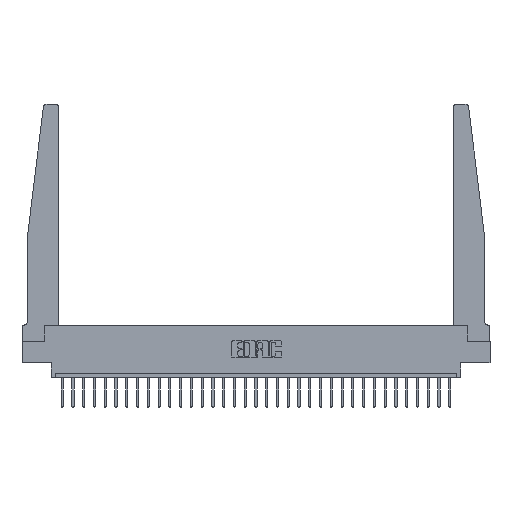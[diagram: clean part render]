
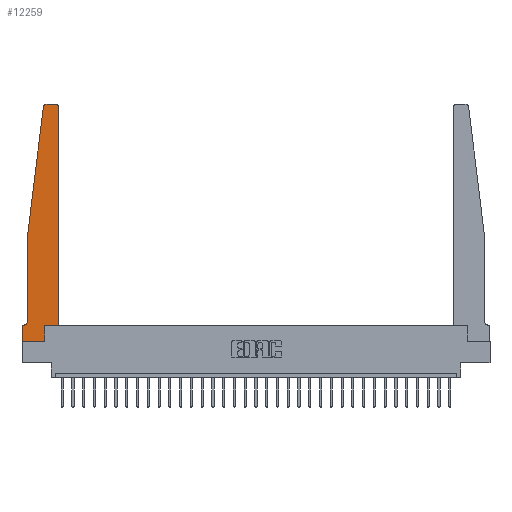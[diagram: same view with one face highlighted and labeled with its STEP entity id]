
A CAD part, top view. The second image highlights one B-rep face of the part: STEP entity #12259.
In plain terms, the highlighted planar face has unit normal (0, 0, 1).
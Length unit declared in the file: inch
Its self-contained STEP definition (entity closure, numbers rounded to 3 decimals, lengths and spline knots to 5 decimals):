
#752 = VERTEX_POINT ( 'NONE', #10985 ) ;
#1044 = CARTESIAN_POINT ( 'NONE',  ( 0.065, 1.25, 0.37 ) ) ;
#1066 = CARTESIAN_POINT ( 'NONE',  ( 0.2605, 0.18, 0.37 ) ) ;
#1808 = DIRECTION ( 'NONE',  ( 1., 0., 0. ) ) ;
#1950 = CARTESIAN_POINT ( 'NONE',  ( 0.395, 2.75, 0.37 ) ) ;
#2526 = DIRECTION ( 'NONE',  ( -1., 0., 0. ) ) ;
#2710 = ORIENTED_EDGE ( 'NONE', *, *, #28389, .T. ) ;
#3268 = CARTESIAN_POINT ( 'NONE',  ( 0.27653, 2.75, 0.37 ) ) ;
#3330 = VERTEX_POINT ( 'NONE', #6117 ) ;
#3364 = LINE ( 'NONE', #13726, #3900 ) ;
#3491 = CARTESIAN_POINT ( 'NONE',  ( 0.065, 0.2375, 0.37 ) ) ;
#3594 = CARTESIAN_POINT ( 'NONE',  ( 0.425, 0.18, 0.37 ) ) ;
#3679 = LINE ( 'NONE', #14845, #21138 ) ;
#3706 = EDGE_CURVE ( 'NONE', #10774, #10416, #12161, .T. ) ;
#3900 = VECTOR ( 'NONE', #22688, 39.37008 ) ;
#4049 = VECTOR ( 'NONE', #21246, 39.37008 ) ;
#4545 = CARTESIAN_POINT ( 'NONE',  ( 0.25, 2.75, 0.37 ) ) ;
#5401 = DIRECTION ( 'NONE',  ( 1., 0., 0. ) ) ;
#5425 = VERTEX_POINT ( 'NONE', #17508 ) ;
#5815 = ORIENTED_EDGE ( 'NONE', *, *, #12716, .T. ) ;
#6117 = CARTESIAN_POINT ( 'NONE',  ( 0.2605, 0.18, 0.37 ) ) ;
#6960 = ORIENTED_EDGE ( 'NONE', *, *, #20712, .T. ) ;
#7152 = VERTEX_POINT ( 'NONE', #1950 ) ;
#7187 = EDGE_CURVE ( 'NONE', #3330, #15897, #26473, .T. ) ;
#7619 = PLANE ( 'NONE',  #15195 ) ;
#7924 = CARTESIAN_POINT ( 'NONE',  ( 0.065, 1.25, 0.37 ) ) ;
#7941 = DIRECTION ( 'NONE',  ( -1., 0., 0. ) ) ;
#7980 = DIRECTION ( 'NONE',  ( 0., 1., 0. ) ) ;
#8244 = ORIENTED_EDGE ( 'NONE', *, *, #13116, .T. ) ;
#8629 = CARTESIAN_POINT ( 'NONE',  ( 0.27653, 2.72, 0.37 ) ) ;
#8886 = EDGE_CURVE ( 'NONE', #5425, #3330, #23819, .T. ) ;
#9019 = EDGE_CURVE ( 'NONE', #15897, #752, #21089, .T. ) ;
#9147 = VERTEX_POINT ( 'NONE', #22843 ) ;
#9743 = CARTESIAN_POINT ( 'NONE',  ( 0., 0., 0.37 ) ) ;
#9792 = ORIENTED_EDGE ( 'NONE', *, *, #3706, .T. ) ;
#10229 = CARTESIAN_POINT ( 'NONE',  ( 0.425, 0.18, 0.37 ) ) ;
#10416 = VERTEX_POINT ( 'NONE', #3491 ) ;
#10774 = VERTEX_POINT ( 'NONE', #15992 ) ;
#10856 = ORIENTED_EDGE ( 'NONE', *, *, #8886, .T. ) ;
#10985 = CARTESIAN_POINT ( 'NONE',  ( 0.425, 2.72, 0.37 ) ) ;
#11043 = CARTESIAN_POINT ( 'NONE',  ( 0.425, 0.18, 0.37 ) ) ;
#11393 = CIRCLE ( 'NONE', #27813, 0.05 ) ;
#11712 = AXIS2_PLACEMENT_3D ( 'NONE', #8629, #24461, #13454 ) ;
#12112 = DIRECTION ( 'NONE',  ( -1., 0., 0. ) ) ;
#12161 = LINE ( 'NONE', #7924, #4049 ) ;
#12259 = ADVANCED_FACE ( 'NONE', ( #27716 ), #7619, .T. ) ;
#12396 = VECTOR ( 'NONE', #24086, 39.37008 ) ;
#12489 = DIRECTION ( 'NONE',  ( 0., 0., 1. ) ) ;
#12716 = EDGE_CURVE ( 'NONE', #9147, #10774, #26163, .T. ) ;
#12717 = AXIS2_PLACEMENT_3D ( 'NONE', #23634, #12489, #23192 ) ;
#13116 = EDGE_CURVE ( 'NONE', #19179, #22123, #23379, .T. ) ;
#13243 = VECTOR ( 'NONE', #27735, 39.37008 ) ;
#13454 = DIRECTION ( 'NONE',  ( 1., 0., 0. ) ) ;
#13726 = CARTESIAN_POINT ( 'NONE',  ( 0., 0., 0.37 ) ) ;
#14601 = CIRCLE ( 'NONE', #12717, 0.03 ) ;
#14845 = CARTESIAN_POINT ( 'NONE',  ( 0.065, 0.1875, 0.37 ) ) ;
#15195 = AXIS2_PLACEMENT_3D ( 'NONE', #16525, #25500, #5401 ) ;
#15259 = VERTEX_POINT ( 'NONE', #3268 ) ;
#15888 = DIRECTION ( 'NONE',  ( 0., 0., -1. ) ) ;
#15897 = VERTEX_POINT ( 'NONE', #11043 ) ;
#15992 = CARTESIAN_POINT ( 'NONE',  ( 0.065, 1.25, 0.37 ) ) ;
#16525 = CARTESIAN_POINT ( 'NONE',  ( 0., 0.1875, 0.37 ) ) ;
#16642 = DIRECTION ( 'NONE',  ( 0., -1., 0. ) ) ;
#16828 = ORIENTED_EDGE ( 'NONE', *, *, #24704, .T. ) ;
#17469 = VECTOR ( 'NONE', #12112, 39.37008 ) ;
#17508 = CARTESIAN_POINT ( 'NONE',  ( 0.2605, 0., 0.37 ) ) ;
#17683 = VECTOR ( 'NONE', #1808, 39.37008 ) ;
#18280 = EDGE_LOOP ( 'NONE', ( #19956, #16828, #5815, #9792, #6960, #19572, #8244, #2710, #10856, #19670, #24414, #28059 ) ) ;
#18804 = EDGE_CURVE ( 'NONE', #752, #7152, #14601, .T. ) ;
#19150 = CARTESIAN_POINT ( 'NONE',  ( 0., 0., 0.37 ) ) ;
#19179 = VERTEX_POINT ( 'NONE', #22192 ) ;
#19572 = ORIENTED_EDGE ( 'NONE', *, *, #26651, .T. ) ;
#19670 = ORIENTED_EDGE ( 'NONE', *, *, #7187, .T. ) ;
#19956 = ORIENTED_EDGE ( 'NONE', *, *, #20917, .T. ) ;
#20264 = VERTEX_POINT ( 'NONE', #25290 ) ;
#20712 = EDGE_CURVE ( 'NONE', #10416, #20264, #11393, .T. ) ;
#20917 = EDGE_CURVE ( 'NONE', #7152, #15259, #27701, .T. ) ;
#21089 = LINE ( 'NONE', #10229, #13243 ) ;
#21138 = VECTOR ( 'NONE', #7941, 39.37008 ) ;
#21246 = DIRECTION ( 'NONE',  ( 0., -1., 0. ) ) ;
#22123 = VERTEX_POINT ( 'NONE', #19150 ) ;
#22192 = CARTESIAN_POINT ( 'NONE',  ( 0., 0.1875, 0.37 ) ) ;
#22688 = DIRECTION ( 'NONE',  ( 1., 0., 0. ) ) ;
#22843 = CARTESIAN_POINT ( 'NONE',  ( 0.24675, 2.72367, 0.37 ) ) ;
#23192 = DIRECTION ( 'NONE',  ( 1., 0., 0. ) ) ;
#23379 = LINE ( 'NONE', #9743, #28380 ) ;
#23634 = CARTESIAN_POINT ( 'NONE',  ( 0.395, 2.72, 0.37 ) ) ;
#23819 = LINE ( 'NONE', #1066, #24031 ) ;
#24031 = VECTOR ( 'NONE', #7980, 39.37008 ) ;
#24086 = DIRECTION ( 'NONE',  ( -0.122, -0.992, 0. ) ) ;
#24327 = CIRCLE ( 'NONE', #11712, 0.03 ) ;
#24414 = ORIENTED_EDGE ( 'NONE', *, *, #9019, .T. ) ;
#24461 = DIRECTION ( 'NONE',  ( 0., 0., 1. ) ) ;
#24704 = EDGE_CURVE ( 'NONE', #15259, #9147, #24327, .T. ) ;
#25251 = CARTESIAN_POINT ( 'NONE',  ( 0.015, 0.2375, 0.37 ) ) ;
#25290 = CARTESIAN_POINT ( 'NONE',  ( 0.015, 0.1875, 0.37 ) ) ;
#25500 = DIRECTION ( 'NONE',  ( 0., 0., 1. ) ) ;
#26163 = LINE ( 'NONE', #1044, #12396 ) ;
#26473 = LINE ( 'NONE', #3594, #17683 ) ;
#26651 = EDGE_CURVE ( 'NONE', #20264, #19179, #3679, .T. ) ;
#27701 = LINE ( 'NONE', #4545, #17469 ) ;
#27716 = FACE_OUTER_BOUND ( 'NONE', #18280, .T. ) ;
#27735 = DIRECTION ( 'NONE',  ( 0., 1., 0. ) ) ;
#27813 = AXIS2_PLACEMENT_3D ( 'NONE', #25251, #15888, #2526 ) ;
#28059 = ORIENTED_EDGE ( 'NONE', *, *, #18804, .T. ) ;
#28380 = VECTOR ( 'NONE', #16642, 39.37008 ) ;
#28389 = EDGE_CURVE ( 'NONE', #22123, #5425, #3364, .T. ) ;
